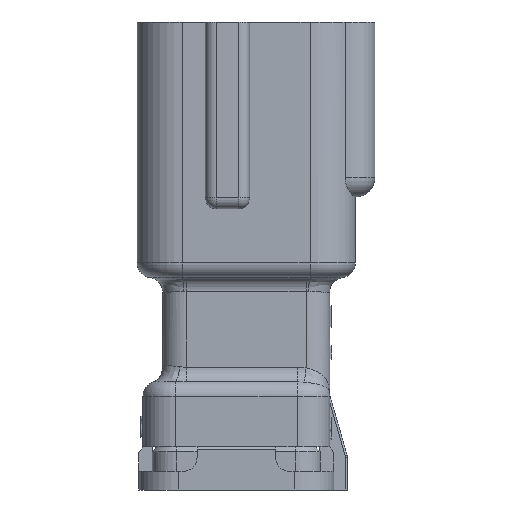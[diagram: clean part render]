
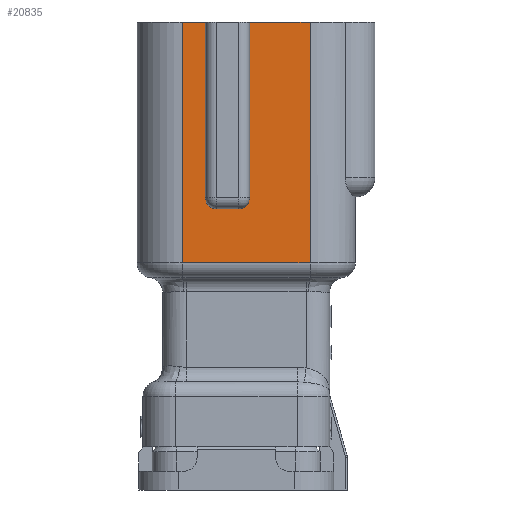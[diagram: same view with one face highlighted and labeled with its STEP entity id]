
A CAD part, left-side view. The second image highlights one B-rep face of the part: STEP entity #20835.
In plain terms, the highlighted planar face has unit normal (-1, 0, 0).
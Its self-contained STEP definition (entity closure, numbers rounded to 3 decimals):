
#80 = DIRECTION ( 'NONE',  ( 0., 0., 1. ) ) ;
#4849 = LINE ( 'NONE', #36923, #23637 ) ;
#5667 = LINE ( 'NONE', #8803, #34037 ) ;
#6042 = DIRECTION ( 'NONE',  ( 0., 1., 0. ) ) ;
#6063 = CARTESIAN_POINT ( 'NONE',  ( -6.911, 1.642, 2.575 ) ) ;
#6598 = CIRCLE ( 'NONE', #14927, 0.55 ) ;
#7013 = VERTEX_POINT ( 'NONE', #17704 ) ;
#7498 = LINE ( 'NONE', #46904, #14270 ) ;
#7708 = CARTESIAN_POINT ( 'NONE',  ( -6.911, 1.092, 2.025 ) ) ;
#8289 = ORIENTED_EDGE ( 'NONE', *, *, #34503, .F. ) ;
#8495 = DIRECTION ( 'NONE',  ( 0., -1., 0. ) ) ;
#8625 = EDGE_CURVE ( 'NONE', #7013, #18116, #41749, .T. ) ;
#8803 = CARTESIAN_POINT ( 'NONE',  ( -6.911, 6.817, 11.525 ) ) ;
#10815 = CARTESIAN_POINT ( 'NONE',  ( -6.911, 1.092, 11.525 ) ) ;
#10825 = LINE ( 'NONE', #38463, #34997 ) ;
#11122 = EDGE_CURVE ( 'NONE', #44859, #44540, #21567, .T. ) ;
#12576 = EDGE_CURVE ( 'NONE', #17943, #49808, #4849, .T. ) ;
#12817 = EDGE_CURVE ( 'NONE', #49808, #44540, #43134, .T. ) ;
#13126 = DIRECTION ( 'NONE',  ( 1., 0., 0. ) ) ;
#13705 = ORIENTED_EDGE ( 'NONE', *, *, #11122, .F. ) ;
#14270 = VECTOR ( 'NONE', #39057, 1000. ) ;
#14748 = EDGE_CURVE ( 'NONE', #42190, #7013, #35373, .T. ) ;
#14927 = AXIS2_PLACEMENT_3D ( 'NONE', #50383, #22718, #38626 ) ;
#15235 = CARTESIAN_POINT ( 'NONE',  ( -6.911, -1.983, -1.475 ) ) ;
#15739 = AXIS2_PLACEMENT_3D ( 'NONE', #31820, #31567, #20072 ) ;
#16983 = VERTEX_POINT ( 'NONE', #32488 ) ;
#17704 = CARTESIAN_POINT ( 'NONE',  ( -6.911, 1.642, 2.025 ) ) ;
#17943 = VERTEX_POINT ( 'NONE', #28977 ) ;
#18116 = VERTEX_POINT ( 'NONE', #21927 ) ;
#20072 = DIRECTION ( 'NONE',  ( 0., 0., 1. ) ) ;
#20418 = CARTESIAN_POINT ( 'NONE',  ( -6.911, 3.342, 11.525 ) ) ;
#20797 = EDGE_CURVE ( 'NONE', #18116, #16983, #6598, .T. ) ;
#20835 = ADVANCED_FACE ( 'NONE', ( #43562 ), #24762, .T. ) ;
#21347 = EDGE_CURVE ( 'NONE', #50074, #17943, #10825, .T. ) ;
#21559 = DIRECTION ( 'NONE',  ( 0., -1., 0. ) ) ;
#21567 = LINE ( 'NONE', #41904, #46053 ) ;
#21927 = CARTESIAN_POINT ( 'NONE',  ( -6.911, 2.792, 2.025 ) ) ;
#22718 = DIRECTION ( 'NONE',  ( 1., 0., 0. ) ) ;
#23177 = ORIENTED_EDGE ( 'NONE', *, *, #21347, .T. ) ;
#23316 = VECTOR ( 'NONE', #51273, 1000. ) ;
#23345 = CARTESIAN_POINT ( 'NONE',  ( -6.911, -1.983, -0.725 ) ) ;
#23637 = VECTOR ( 'NONE', #8495, 1000. ) ;
#23690 = EDGE_LOOP ( 'NONE', ( #23177, #29391, #32618, #13705, #8289, #43131, #31794, #37065, #33858, #24307 ) ) ;
#23866 = LINE ( 'NONE', #7708, #23316 ) ;
#24307 = ORIENTED_EDGE ( 'NONE', *, *, #33268, .F. ) ;
#24540 = EDGE_CURVE ( 'NONE', #16983, #42991, #7498, .T. ) ;
#24762 = PLANE ( 'NONE',  #15739 ) ;
#25091 = DIRECTION ( 'NONE',  ( 0., 0., 1. ) ) ;
#26159 = VECTOR ( 'NONE', #80, 1000. ) ;
#28977 = CARTESIAN_POINT ( 'NONE',  ( -6.911, 4.517, -0.725 ) ) ;
#29391 = ORIENTED_EDGE ( 'NONE', *, *, #12576, .T. ) ;
#31567 = DIRECTION ( 'NONE',  ( -1., 0., 0. ) ) ;
#31794 = ORIENTED_EDGE ( 'NONE', *, *, #8625, .T. ) ;
#31820 = CARTESIAN_POINT ( 'NONE',  ( -6.911, 6.817, -1.475 ) ) ;
#32488 = CARTESIAN_POINT ( 'NONE',  ( -6.911, 3.342, 2.575 ) ) ;
#32618 = ORIENTED_EDGE ( 'NONE', *, *, #12817, .T. ) ;
#33268 = EDGE_CURVE ( 'NONE', #50074, #42991, #5667, .T. ) ;
#33858 = ORIENTED_EDGE ( 'NONE', *, *, #24540, .T. ) ;
#34037 = VECTOR ( 'NONE', #21559, 1000. ) ;
#34503 = EDGE_CURVE ( 'NONE', #42190, #44859, #23866, .T. ) ;
#34997 = VECTOR ( 'NONE', #42636, 1000. ) ;
#35373 = CIRCLE ( 'NONE', #46232, 0.55 ) ;
#35379 = CARTESIAN_POINT ( 'NONE',  ( -6.911, -1.983, 11.525 ) ) ;
#36014 = CARTESIAN_POINT ( 'NONE',  ( -6.911, 4.517, 11.525 ) ) ;
#36923 = CARTESIAN_POINT ( 'NONE',  ( -6.911, -1.983, -0.725 ) ) ;
#36970 = CARTESIAN_POINT ( 'NONE',  ( -6.911, 1.092, 2.575 ) ) ;
#37065 = ORIENTED_EDGE ( 'NONE', *, *, #20797, .T. ) ;
#38099 = CARTESIAN_POINT ( 'NONE',  ( -6.911, 3.342, 2.025 ) ) ;
#38463 = CARTESIAN_POINT ( 'NONE',  ( -6.911, 4.517, -1.475 ) ) ;
#38626 = DIRECTION ( 'NONE',  ( 0., 0., 1. ) ) ;
#39057 = DIRECTION ( 'NONE',  ( 0., 0., 1. ) ) ;
#41749 = LINE ( 'NONE', #38099, #42805 ) ;
#41904 = CARTESIAN_POINT ( 'NONE',  ( -6.911, 6.817, 11.525 ) ) ;
#42190 = VERTEX_POINT ( 'NONE', #36970 ) ;
#42636 = DIRECTION ( 'NONE',  ( 0., 0., -1. ) ) ;
#42805 = VECTOR ( 'NONE', #6042, 1000. ) ;
#42991 = VERTEX_POINT ( 'NONE', #20418 ) ;
#43131 = ORIENTED_EDGE ( 'NONE', *, *, #14748, .T. ) ;
#43134 = LINE ( 'NONE', #15235, #26159 ) ;
#43562 = FACE_OUTER_BOUND ( 'NONE', #23690, .T. ) ;
#44540 = VERTEX_POINT ( 'NONE', #35379 ) ;
#44859 = VERTEX_POINT ( 'NONE', #10815 ) ;
#45588 = DIRECTION ( 'NONE',  ( 0., -1., 0. ) ) ;
#46053 = VECTOR ( 'NONE', #45588, 1000. ) ;
#46232 = AXIS2_PLACEMENT_3D ( 'NONE', #6063, #13126, #25091 ) ;
#46904 = CARTESIAN_POINT ( 'NONE',  ( -6.911, 3.342, 2.025 ) ) ;
#49808 = VERTEX_POINT ( 'NONE', #23345 ) ;
#50074 = VERTEX_POINT ( 'NONE', #36014 ) ;
#50383 = CARTESIAN_POINT ( 'NONE',  ( -6.911, 2.792, 2.575 ) ) ;
#51273 = DIRECTION ( 'NONE',  ( 0., 0., 1. ) ) ;
